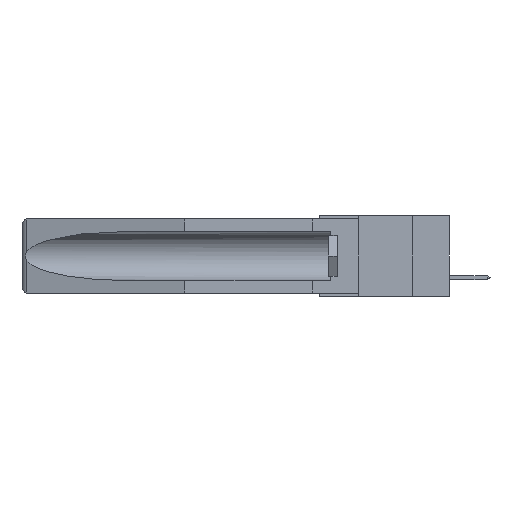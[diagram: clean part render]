
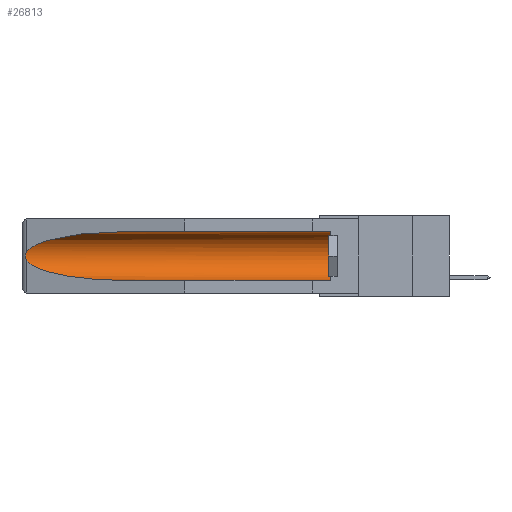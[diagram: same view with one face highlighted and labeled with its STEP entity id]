
A CAD part, left-side view. The second image highlights one B-rep face of the part: STEP entity #26813.
In plain terms, the highlighted cylindrical face has radius 2.857 mm (diameter 5.715 mm), a partial arc.
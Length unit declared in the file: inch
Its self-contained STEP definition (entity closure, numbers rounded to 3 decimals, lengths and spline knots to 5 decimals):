
#808 = CARTESIAN_POINT ( 'NONE',  ( 0.155, -0.30754, -0.059 ) ) ;
#1086 = CARTESIAN_POINT ( 'NONE',  ( 0.26655, 1.53094, -0.18657 ) ) ;
#1517 = EDGE_CURVE ( 'NONE', #20013, #13633, #2955, .T. ) ;
#2722 = FACE_OUTER_BOUND ( 'NONE', #24309, .T. ) ;
#2955 =( BOUNDED_CURVE ( )  B_SPLINE_CURVE ( 3, ( #14494, #19235, #27063, #24724 ),
 .UNSPECIFIED., .F., .F. ) 
 B_SPLINE_CURVE_WITH_KNOTS ( ( 4, 4 ),
 ( 0.1948, 1.5708 ),
 .UNSPECIFIED. ) 
 CURVE ( )  GEOMETRIC_REPRESENTATION_ITEM ( )  RATIONAL_B_SPLINE_CURVE ( ( 1., 0.848, 0.848, 1. ) ) 
 REPRESENTATION_ITEM ( '' )  );
#4286 = CARTESIAN_POINT ( 'NONE',  ( 0.26537, 1.52718, -0.14972 ) ) ;
#4343 = CARTESIAN_POINT ( 'NONE',  ( 0.155, -0.30754, -0.1715 ) ) ;
#4527 = CARTESIAN_POINT ( 'NONE',  ( 0.155, 1.07973, -0.059 ) ) ;
#4881 = CARTESIAN_POINT ( 'NONE',  ( 0.155, 0.126, -0.059 ) ) ;
#4922 = DIRECTION ( 'NONE',  ( 0., -1., 0. ) ) ;
#5323 = AXIS2_PLACEMENT_3D ( 'NONE', #7767, #4922, #25317 ) ;
#5490 = EDGE_CURVE ( 'NONE', #22946, #18111, #25390, .T. ) ;
#5774 = ORIENTED_EDGE ( 'NONE', *, *, #16763, .T. ) ;
#5998 = CARTESIAN_POINT ( 'NONE',  ( 0.155, -0.30754, -0.284 ) ) ;
#6185 = CIRCLE ( 'NONE', #5323, 0.1125 ) ;
#7229 = CARTESIAN_POINT ( 'NONE',  ( 0.26537, 1.52718, -0.14972 ) ) ;
#7767 = CARTESIAN_POINT ( 'NONE',  ( 0.155, 0.126, -0.1715 ) ) ;
#8605 = CARTESIAN_POINT ( 'NONE',  ( 0.26654, 1.53092, -0.15636 ) ) ;
#8819 = CARTESIAN_POINT ( 'NONE',  ( 0.2673, 1.5327, -0.16383 ) ) ;
#8830 = ORIENTED_EDGE ( 'NONE', *, *, #1517, .T. ) ;
#9461 = CARTESIAN_POINT ( 'NONE',  ( 0.25451, 1.48313, -0.09465 ) ) ;
#9672 = CARTESIAN_POINT ( 'NONE',  ( 0.155, 1.07973, -0.059 ) ) ;
#10037 = EDGE_CURVE ( 'NONE', #18111, #20013, #18119, .T. ) ;
#10556 = ORIENTED_EDGE ( 'NONE', *, *, #5490, .T. ) ;
#10653 = ORIENTED_EDGE ( 'NONE', *, *, #15606, .F. ) ;
#11541 = EDGE_CURVE ( 'NONE', #31819, #25052, #6185, .T. ) ;
#11896 = CARTESIAN_POINT ( 'NONE',  ( 0.21114, 1.30732, -0.059 ) ) ;
#13348 = ORIENTED_EDGE ( 'NONE', *, *, #10037, .T. ) ;
#13588 = DIRECTION ( 'NONE',  ( 0., 1., 0. ) ) ;
#13633 = VERTEX_POINT ( 'NONE', #25354 ) ;
#13699 = LINE ( 'NONE', #808, #29892 ) ;
#13743 = ORIENTED_EDGE ( 'NONE', *, *, #11541, .T. ) ;
#14494 = CARTESIAN_POINT ( 'NONE',  ( 0.26537, 1.52718, -0.19328 ) ) ;
#14795 = DIRECTION ( 'NONE',  ( 0., 1., 0. ) ) ;
#14821 = AXIS2_PLACEMENT_3D ( 'NONE', #4343, #14795, #21947 ) ;
#15127 = CARTESIAN_POINT ( 'NONE',  ( 0.26537, 1.52718, -0.14972 ) ) ;
#15606 = EDGE_CURVE ( 'NONE', #31819, #13633, #17654, .T. ) ;
#16414 = CARTESIAN_POINT ( 'NONE',  ( 0.2675, 1.53308, -0.17534 ) ) ;
#16763 = EDGE_CURVE ( 'NONE', #25052, #22946, #13699, .T. ) ;
#17654 = LINE ( 'NONE', #5998, #20810 ) ;
#18111 = VERTEX_POINT ( 'NONE', #15127 ) ;
#18119 = B_SPLINE_CURVE_WITH_KNOTS ( 'NONE', 3,
 ( #7229, #18839, #8605, #8819, #23583, #16414, #31297, #1086, #28797, #26468 ),
 .UNSPECIFIED., .F., .F.,
 ( 4, 2, 2, 2, 4 ),
 ( 0., 0.00029, 0.00058, 0.00087, 0.00117 ),
 .UNSPECIFIED. ) ;
#18839 = CARTESIAN_POINT ( 'NONE',  ( 0.26597, 1.52961, -0.15275 ) ) ;
#19235 = CARTESIAN_POINT ( 'NONE',  ( 0.25451, 1.48313, -0.24835 ) ) ;
#20013 = VERTEX_POINT ( 'NONE', #29466 ) ;
#20810 = VECTOR ( 'NONE', #30823, 39.37008 ) ;
#21947 = DIRECTION ( 'NONE',  ( 0., 0., 1. ) ) ;
#22946 = VERTEX_POINT ( 'NONE', #4527 ) ;
#23583 = CARTESIAN_POINT ( 'NONE',  ( 0.2675, 1.53308, -0.16763 ) ) ;
#23728 = CARTESIAN_POINT ( 'NONE',  ( 0.155, 0.126, -0.284 ) ) ;
#24309 = EDGE_LOOP ( 'NONE', ( #10556, #13348, #8830, #10653, #13743, #5774 ) ) ;
#24724 = CARTESIAN_POINT ( 'NONE',  ( 0.155, 1.07973, -0.284 ) ) ;
#25052 = VERTEX_POINT ( 'NONE', #4881 ) ;
#25317 = DIRECTION ( 'NONE',  ( 0., 0., 1. ) ) ;
#25354 = CARTESIAN_POINT ( 'NONE',  ( 0.155, 1.07973, -0.284 ) ) ;
#25390 =( BOUNDED_CURVE ( )  B_SPLINE_CURVE ( 3, ( #9672, #11896, #9461, #4286 ),
 .UNSPECIFIED., .F., .F. ) 
 B_SPLINE_CURVE_WITH_KNOTS ( ( 4, 4 ),
 ( 4.71239, 6.08839 ),
 .UNSPECIFIED. ) 
 CURVE ( )  GEOMETRIC_REPRESENTATION_ITEM ( )  RATIONAL_B_SPLINE_CURVE ( ( 1., 0.848, 0.848, 1. ) ) 
 REPRESENTATION_ITEM ( '' )  );
#26468 = CARTESIAN_POINT ( 'NONE',  ( 0.26537, 1.52718, -0.19328 ) ) ;
#26813 = ADVANCED_FACE ( 'NONE', ( #2722 ), #27170, .F. ) ;
#27063 = CARTESIAN_POINT ( 'NONE',  ( 0.21114, 1.30732, -0.284 ) ) ;
#27170 = CYLINDRICAL_SURFACE ( 'NONE', #14821, 0.1125 ) ;
#28797 = CARTESIAN_POINT ( 'NONE',  ( 0.26597, 1.5296, -0.19026 ) ) ;
#29466 = CARTESIAN_POINT ( 'NONE',  ( 0.26537, 1.52718, -0.19328 ) ) ;
#29892 = VECTOR ( 'NONE', #13588, 39.37008 ) ;
#30823 = DIRECTION ( 'NONE',  ( 0., 1., 0. ) ) ;
#31297 = CARTESIAN_POINT ( 'NONE',  ( 0.2673, 1.53269, -0.17917 ) ) ;
#31819 = VERTEX_POINT ( 'NONE', #23728 ) ;
